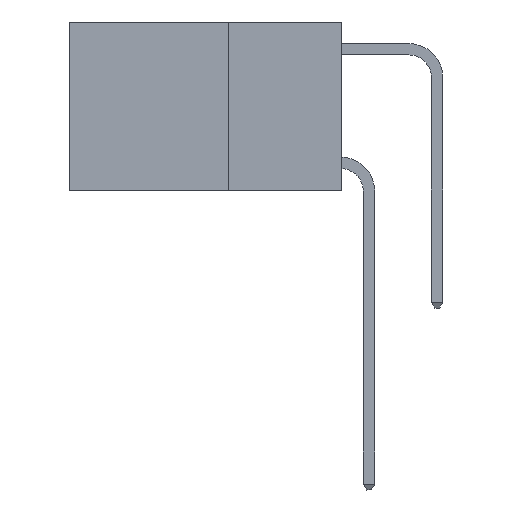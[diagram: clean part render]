
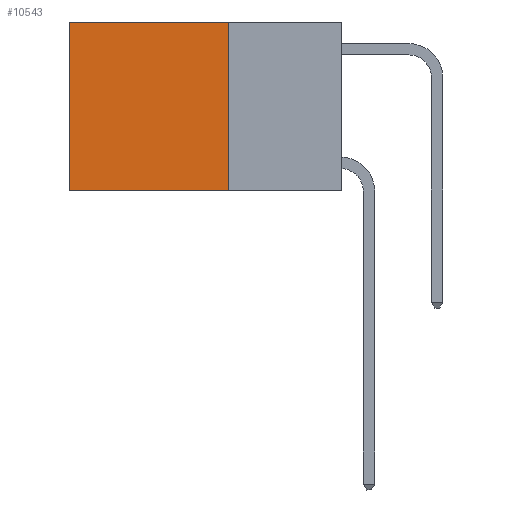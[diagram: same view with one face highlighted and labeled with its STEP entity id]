
A CAD part, left-side view. The second image highlights one B-rep face of the part: STEP entity #10543.
In plain terms, the highlighted planar face has unit normal (-1, 0, 0).
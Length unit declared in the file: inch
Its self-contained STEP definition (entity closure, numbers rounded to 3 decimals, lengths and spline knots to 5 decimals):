
#314 = VECTOR ( 'NONE', #9723, 39.37008 ) ;
#496 = VERTEX_POINT ( 'NONE', #4077 ) ;
#513 = LINE ( 'NONE', #5407, #9726 ) ;
#832 = DIRECTION ( 'NONE',  ( 1., 0., 0. ) ) ;
#1674 = VECTOR ( 'NONE', #9353, 39.37008 ) ;
#1765 = EDGE_CURVE ( 'NONE', #3064, #4145, #513, .T. ) ;
#2817 = CARTESIAN_POINT ( 'NONE',  ( 0.2625, 0.6, 0. ) ) ;
#3064 = VERTEX_POINT ( 'NONE', #2817 ) ;
#3670 = CARTESIAN_POINT ( 'NONE',  ( 0.2625, 0.25, 0. ) ) ;
#3728 = ORIENTED_EDGE ( 'NONE', *, *, #1765, .T. ) ;
#4077 = CARTESIAN_POINT ( 'NONE',  ( 0.2625, 0.25, -0.37 ) ) ;
#4145 = VERTEX_POINT ( 'NONE', #7091 ) ;
#5154 = EDGE_LOOP ( 'NONE', ( #3728, #11776, #12171, #9446 ) ) ;
#5407 = CARTESIAN_POINT ( 'NONE',  ( 0.2625, 0.6, 0. ) ) ;
#5542 = DIRECTION ( 'NONE',  ( 0., 1., 0. ) ) ;
#7077 = EDGE_CURVE ( 'NONE', #496, #4145, #11523, .T. ) ;
#7091 = CARTESIAN_POINT ( 'NONE',  ( 0.2625, 0.6, -0.37 ) ) ;
#7128 = EDGE_CURVE ( 'NONE', #12797, #496, #12643, .T. ) ;
#7422 = CARTESIAN_POINT ( 'NONE',  ( 0.2625, 0.25, 0. ) ) ;
#7456 = CARTESIAN_POINT ( 'NONE',  ( 0.2625, 0.25, -0.37 ) ) ;
#7611 = CARTESIAN_POINT ( 'NONE',  ( 0.2625, 0.25, 0. ) ) ;
#8509 = LINE ( 'NONE', #7611, #1674 ) ;
#8808 = DIRECTION ( 'NONE',  ( 0., 0., -1. ) ) ;
#9026 = PLANE ( 'NONE',  #11887 ) ;
#9045 = VECTOR ( 'NONE', #5542, 39.37008 ) ;
#9332 = EDGE_CURVE ( 'NONE', #12797, #3064, #8509, .T. ) ;
#9353 = DIRECTION ( 'NONE',  ( 0., 1., 0. ) ) ;
#9446 = ORIENTED_EDGE ( 'NONE', *, *, #9332, .T. ) ;
#9470 = DIRECTION ( 'NONE',  ( 0., 0., -1. ) ) ;
#9649 = CARTESIAN_POINT ( 'NONE',  ( 0.2625, 0.25, 0. ) ) ;
#9723 = DIRECTION ( 'NONE',  ( 0., 0., -1. ) ) ;
#9726 = VECTOR ( 'NONE', #9470, 39.37008 ) ;
#9837 = FACE_OUTER_BOUND ( 'NONE', #5154, .T. ) ;
#10543 = ADVANCED_FACE ( 'NONE', ( #9837 ), #9026, .F. ) ;
#11523 = LINE ( 'NONE', #7456, #9045 ) ;
#11776 = ORIENTED_EDGE ( 'NONE', *, *, #7077, .F. ) ;
#11887 = AXIS2_PLACEMENT_3D ( 'NONE', #3670, #832, #8808 ) ;
#12171 = ORIENTED_EDGE ( 'NONE', *, *, #7128, .F. ) ;
#12643 = LINE ( 'NONE', #9649, #314 ) ;
#12797 = VERTEX_POINT ( 'NONE', #7422 ) ;
